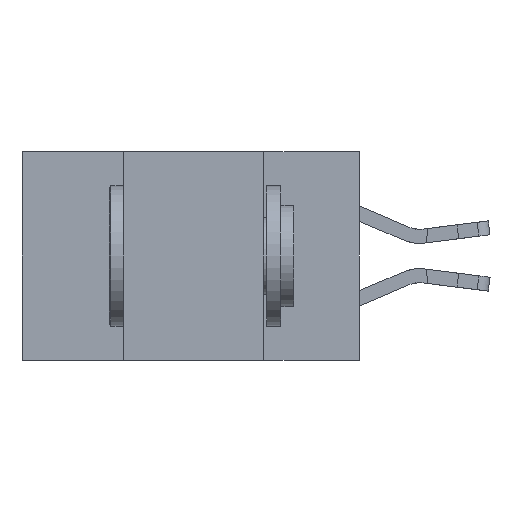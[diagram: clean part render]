
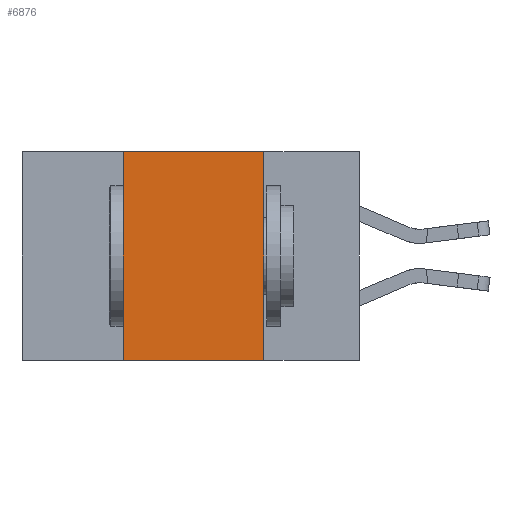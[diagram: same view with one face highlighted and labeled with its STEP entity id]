
A CAD part, left-side view. The second image highlights one B-rep face of the part: STEP entity #6876.
In plain terms, the highlighted planar face has unit normal (-1, 0, 0).
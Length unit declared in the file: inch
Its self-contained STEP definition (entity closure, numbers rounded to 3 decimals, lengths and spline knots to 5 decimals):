
#934 = EDGE_LOOP ( 'NONE', ( #8271, #14659, #8972, #3136 ) ) ;
#1511 = VECTOR ( 'NONE', #16280, 39.37008 ) ;
#2244 = VECTOR ( 'NONE', #12542, 39.37008 ) ;
#2591 = PLANE ( 'NONE',  #3480 ) ;
#2760 = VERTEX_POINT ( 'NONE', #14016 ) ;
#3136 = ORIENTED_EDGE ( 'NONE', *, *, #4619, .T. ) ;
#3480 = AXIS2_PLACEMENT_3D ( 'NONE', #10861, #5522, #14726 ) ;
#3519 = VERTEX_POINT ( 'NONE', #5411 ) ;
#3527 = EDGE_CURVE ( 'NONE', #2760, #14225, #3775, .T. ) ;
#3775 = LINE ( 'NONE', #10699, #10183 ) ;
#4599 = CARTESIAN_POINT ( 'NONE',  ( 0., 0.6, -0.37 ) ) ;
#4619 = EDGE_CURVE ( 'NONE', #2760, #3519, #13211, .T. ) ;
#5411 = CARTESIAN_POINT ( 'NONE',  ( 0., 0.17, -0.37 ) ) ;
#5522 = DIRECTION ( 'NONE',  ( 1., 0., 0. ) ) ;
#6033 = DIRECTION ( 'NONE',  ( 0., -1., 0. ) ) ;
#6812 = CARTESIAN_POINT ( 'NONE',  ( 0., 0.42, 0. ) ) ;
#6876 = ADVANCED_FACE ( 'NONE', ( #10694 ), #2591, .F. ) ;
#8128 = VECTOR ( 'NONE', #6033, 39.37008 ) ;
#8271 = ORIENTED_EDGE ( 'NONE', *, *, #16378, .F. ) ;
#8972 = ORIENTED_EDGE ( 'NONE', *, *, #3527, .F. ) ;
#10183 = VECTOR ( 'NONE', #12004, 39.37008 ) ;
#10393 = VERTEX_POINT ( 'NONE', #15736 ) ;
#10694 = FACE_OUTER_BOUND ( 'NONE', #934, .T. ) ;
#10699 = CARTESIAN_POINT ( 'NONE',  ( 0., 0.42, 0. ) ) ;
#10861 = CARTESIAN_POINT ( 'NONE',  ( 0., 0.6, 0. ) ) ;
#11001 = CARTESIAN_POINT ( 'NONE',  ( 0., 0.17, 0. ) ) ;
#11924 = EDGE_CURVE ( 'NONE', #14225, #10393, #12001, .T. ) ;
#12001 = LINE ( 'NONE', #16747, #8128 ) ;
#12004 = DIRECTION ( 'NONE',  ( 0., 0., 1. ) ) ;
#12482 = LINE ( 'NONE', #11001, #1511 ) ;
#12542 = DIRECTION ( 'NONE',  ( 0., -1., 0. ) ) ;
#13211 = LINE ( 'NONE', #4599, #2244 ) ;
#14016 = CARTESIAN_POINT ( 'NONE',  ( 0., 0.42, -0.37 ) ) ;
#14225 = VERTEX_POINT ( 'NONE', #6812 ) ;
#14659 = ORIENTED_EDGE ( 'NONE', *, *, #11924, .F. ) ;
#14726 = DIRECTION ( 'NONE',  ( 0., 0., -1. ) ) ;
#15736 = CARTESIAN_POINT ( 'NONE',  ( 0., 0.17, 0. ) ) ;
#16280 = DIRECTION ( 'NONE',  ( 0., 0., -1. ) ) ;
#16378 = EDGE_CURVE ( 'NONE', #10393, #3519, #12482, .T. ) ;
#16747 = CARTESIAN_POINT ( 'NONE',  ( 0., 0.6, 0. ) ) ;
